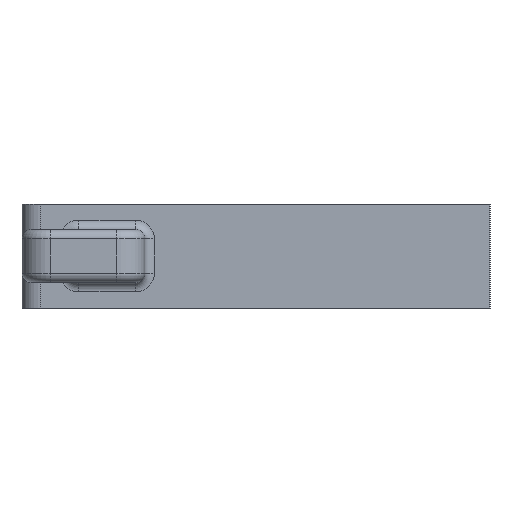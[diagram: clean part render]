
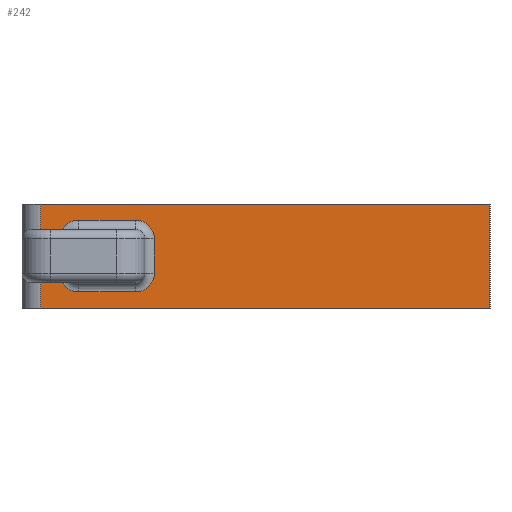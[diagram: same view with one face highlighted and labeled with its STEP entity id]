
A CAD part, front view. The second image highlights one B-rep face of the part: STEP entity #242.
In plain terms, the highlighted planar face has unit normal (0, -1, 0).
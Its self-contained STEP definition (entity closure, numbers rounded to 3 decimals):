
#75=CARTESIAN_POINT('',(2.,11.3,-5.5));
#76=VERTEX_POINT('',#75);
#84=CARTESIAN_POINT('',(2.,11.3,5.5));
#85=VERTEX_POINT('',#84);
#86=CARTESIAN_POINT('',(2.,11.3,-5.5));
#87=DIRECTION('',(0.0,0.0,1.0));
#88=VECTOR('',#87,11.0);
#89=LINE('',#86,#88);
#90=EDGE_CURVE('',#76,#85,#89,.T.);
#116=CARTESIAN_POINT('',(49.5,11.3,5.5));
#117=VERTEX_POINT('',#116);
#118=CARTESIAN_POINT('',(49.5,11.3,5.5));
#119=DIRECTION('',(-1.0,0.0,0.0));
#120=VECTOR('',#119,47.5);
#121=LINE('',#118,#120);
#122=EDGE_CURVE('',#117,#85,#121,.T.);
#149=CARTESIAN_POINT('',(49.5,11.3,0.0));
#150=DIRECTION('',(0.0,-1.0,0.0));
#151=DIRECTION('',(0.0,0.0,-1.0));
#152=AXIS2_PLACEMENT_3D('',#149,#150,#151);
#153=PLANE('',#152);
#154=ORIENTED_EDGE('',*,*,#90,.F.);
#155=CARTESIAN_POINT('',(49.5,11.3,-5.5));
#156=VERTEX_POINT('',#155);
#157=CARTESIAN_POINT('',(2.,11.3,-5.5));
#158=DIRECTION('',(1.0,0.0,0.0));
#159=VECTOR('',#158,47.5);
#160=LINE('',#157,#159);
#161=EDGE_CURVE('',#76,#156,#160,.T.);
#162=ORIENTED_EDGE('',*,*,#161,.T.);
#163=CARTESIAN_POINT('',(49.5,11.3,-5.5));
#164=DIRECTION('',(0.0,0.0,1.0));
#165=VECTOR('',#164,11.0);
#166=LINE('',#163,#165);
#167=EDGE_CURVE('',#156,#117,#166,.T.);
#168=ORIENTED_EDGE('',*,*,#167,.T.);
#169=ORIENTED_EDGE('',*,*,#122,.T.);
#170=EDGE_LOOP('',(#154,#162,#168,#169));
#171=FACE_OUTER_BOUND('',#170,.T.);
#172=CARTESIAN_POINT('',(14.,11.3,1.8));
#173=VERTEX_POINT('',#172);
#174=CARTESIAN_POINT('',(12.,11.3,3.8));
#175=VERTEX_POINT('',#174);
#176=CARTESIAN_POINT('',(12.,11.3,1.8));
#177=DIRECTION('',(0.,-1.0,0.));
#178=DIRECTION('',(0.707,0.,0.707));
#179=AXIS2_PLACEMENT_3D('',#176,#177,#178);
#180=CIRCLE('',#179,2.0);
#181=EDGE_CURVE('',#173,#175,#180,.T.);
#182=ORIENTED_EDGE('',*,*,#181,.F.);
#183=CARTESIAN_POINT('',(14.,11.3,-1.8));
#184=VERTEX_POINT('',#183);
#185=CARTESIAN_POINT('',(14.,11.3,-1.8));
#186=DIRECTION('',(0.0,0.0,1.0));
#187=VECTOR('',#186,3.6);
#188=LINE('',#185,#187);
#189=EDGE_CURVE('',#184,#173,#188,.T.);
#190=ORIENTED_EDGE('',*,*,#189,.F.);
#191=CARTESIAN_POINT('',(12.,11.3,-3.8));
#192=VERTEX_POINT('',#191);
#193=CARTESIAN_POINT('',(12.,11.3,-1.8));
#194=DIRECTION('',(0.,-1.0,0.));
#195=DIRECTION('',(0.707,0.,-0.707));
#196=AXIS2_PLACEMENT_3D('',#193,#194,#195);
#197=CIRCLE('',#196,2.0);
#198=EDGE_CURVE('',#192,#184,#197,.T.);
#199=ORIENTED_EDGE('',*,*,#198,.F.);
#200=CARTESIAN_POINT('',(6.,11.3,-3.8));
#201=VERTEX_POINT('',#200);
#202=CARTESIAN_POINT('',(6.,11.3,-3.8));
#203=DIRECTION('',(1.0,0.0,0.0));
#204=VECTOR('',#203,6.);
#205=LINE('',#202,#204);
#206=EDGE_CURVE('',#201,#192,#205,.T.);
#207=ORIENTED_EDGE('',*,*,#206,.F.);
#208=CARTESIAN_POINT('',(4.,11.3,-1.8));
#209=VERTEX_POINT('',#208);
#210=CARTESIAN_POINT('',(6.,11.3,-1.8));
#211=DIRECTION('',(0.,-1.0,0.));
#212=DIRECTION('',(-0.707,0.,-0.707));
#213=AXIS2_PLACEMENT_3D('',#210,#211,#212);
#214=CIRCLE('',#213,2.0);
#215=EDGE_CURVE('',#209,#201,#214,.T.);
#216=ORIENTED_EDGE('',*,*,#215,.F.);
#217=CARTESIAN_POINT('',(4.,11.3,1.8));
#218=VERTEX_POINT('',#217);
#219=CARTESIAN_POINT('',(4.,11.3,1.8));
#220=DIRECTION('',(0.0,0.0,-1.0));
#221=VECTOR('',#220,3.6);
#222=LINE('',#219,#221);
#223=EDGE_CURVE('',#218,#209,#222,.T.);
#224=ORIENTED_EDGE('',*,*,#223,.F.);
#225=CARTESIAN_POINT('',(6.,11.3,3.8));
#226=VERTEX_POINT('',#225);
#227=CARTESIAN_POINT('',(6.,11.3,1.8));
#228=DIRECTION('',(0.,-1.0,0.));
#229=DIRECTION('',(-0.707,0.,0.707));
#230=AXIS2_PLACEMENT_3D('',#227,#228,#229);
#231=CIRCLE('',#230,2.0);
#232=EDGE_CURVE('',#226,#218,#231,.T.);
#233=ORIENTED_EDGE('',*,*,#232,.F.);
#234=CARTESIAN_POINT('',(12.,11.3,3.8));
#235=DIRECTION('',(-1.0,0.0,0.0));
#236=VECTOR('',#235,6.);
#237=LINE('',#234,#236);
#238=EDGE_CURVE('',#175,#226,#237,.T.);
#239=ORIENTED_EDGE('',*,*,#238,.F.);
#240=EDGE_LOOP('',(#182,#190,#199,#207,#216,#224,#233,#239));
#241=FACE_BOUND('',#240,.T.);
#242=ADVANCED_FACE('',(#171,#241),#153,.T.);
